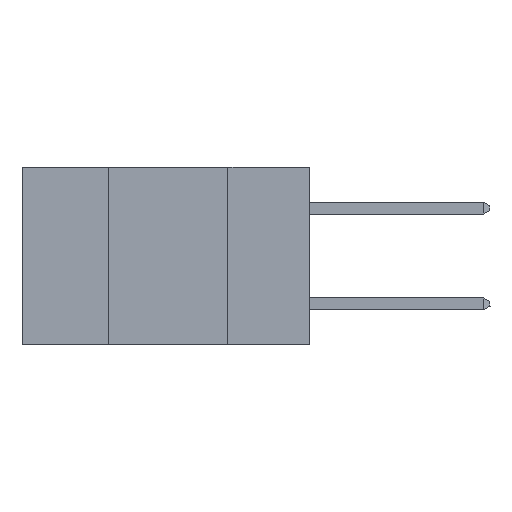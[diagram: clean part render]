
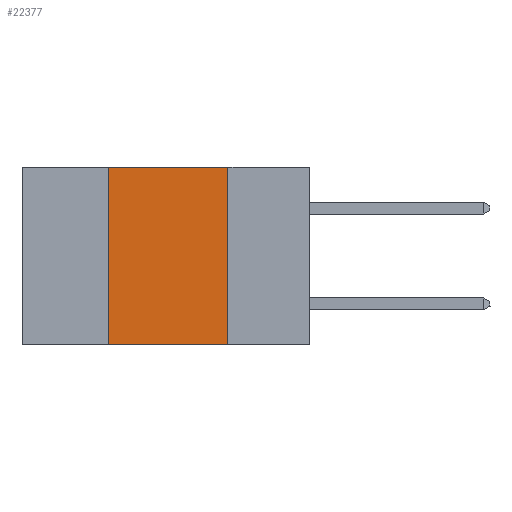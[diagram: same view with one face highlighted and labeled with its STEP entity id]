
A CAD part, left-side view. The second image highlights one B-rep face of the part: STEP entity #22377.
In plain terms, the highlighted planar face has unit normal (-1, 0, 0).
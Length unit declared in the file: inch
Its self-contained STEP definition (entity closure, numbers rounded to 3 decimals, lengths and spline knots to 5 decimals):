
#295 = EDGE_CURVE ( 'NONE', #17158, #25781, #14464, .T. ) ;
#1263 = EDGE_LOOP ( 'NONE', ( #10814, #28822, #29011, #9692 ) ) ;
#1396 = CARTESIAN_POINT ( 'NONE',  ( 0., 0.17, -0.37 ) ) ;
#2312 = VECTOR ( 'NONE', #17650, 39.37008 ) ;
#3037 = AXIS2_PLACEMENT_3D ( 'NONE', #12437, #6831, #18360 ) ;
#5322 = DIRECTION ( 'NONE',  ( 0., -1., 0. ) ) ;
#5806 = LINE ( 'NONE', #28893, #7790 ) ;
#6831 = DIRECTION ( 'NONE',  ( 1., 0., 0. ) ) ;
#7790 = VECTOR ( 'NONE', #18457, 39.37008 ) ;
#9297 = PLANE ( 'NONE',  #3037 ) ;
#9692 = ORIENTED_EDGE ( 'NONE', *, *, #11433, .T. ) ;
#9768 = CARTESIAN_POINT ( 'NONE',  ( 0., 0.6, -0.37 ) ) ;
#10146 = CARTESIAN_POINT ( 'NONE',  ( 0., 0.42, -0.37 ) ) ;
#10175 = CARTESIAN_POINT ( 'NONE',  ( 0., 0.17, 0. ) ) ;
#10814 = ORIENTED_EDGE ( 'NONE', *, *, #295, .F. ) ;
#11433 = EDGE_CURVE ( 'NONE', #31203, #25781, #30678, .T. ) ;
#12437 = CARTESIAN_POINT ( 'NONE',  ( 0., 0.6, 0. ) ) ;
#14464 = LINE ( 'NONE', #10175, #2312 ) ;
#15812 = LINE ( 'NONE', #20394, #26854 ) ;
#17158 = VERTEX_POINT ( 'NONE', #29191 ) ;
#17650 = DIRECTION ( 'NONE',  ( 0., 0., -1. ) ) ;
#18360 = DIRECTION ( 'NONE',  ( 0., 0., -1. ) ) ;
#18442 = EDGE_CURVE ( 'NONE', #31203, #27503, #5806, .T. ) ;
#18457 = DIRECTION ( 'NONE',  ( 0., 0., 1. ) ) ;
#20394 = CARTESIAN_POINT ( 'NONE',  ( 0., 0.6, 0. ) ) ;
#21438 = FACE_OUTER_BOUND ( 'NONE', #1263, .T. ) ;
#22377 = ADVANCED_FACE ( 'NONE', ( #21438 ), #9297, .F. ) ;
#23201 = EDGE_CURVE ( 'NONE', #27503, #17158, #15812, .T. ) ;
#24090 = VECTOR ( 'NONE', #28735, 39.37008 ) ;
#25781 = VERTEX_POINT ( 'NONE', #1396 ) ;
#25930 = CARTESIAN_POINT ( 'NONE',  ( 0., 0.42, 0. ) ) ;
#26854 = VECTOR ( 'NONE', #5322, 39.37008 ) ;
#27503 = VERTEX_POINT ( 'NONE', #25930 ) ;
#28735 = DIRECTION ( 'NONE',  ( 0., -1., 0. ) ) ;
#28822 = ORIENTED_EDGE ( 'NONE', *, *, #23201, .F. ) ;
#28893 = CARTESIAN_POINT ( 'NONE',  ( 0., 0.42, 0. ) ) ;
#29011 = ORIENTED_EDGE ( 'NONE', *, *, #18442, .F. ) ;
#29191 = CARTESIAN_POINT ( 'NONE',  ( 0., 0.17, 0. ) ) ;
#30678 = LINE ( 'NONE', #9768, #24090 ) ;
#31203 = VERTEX_POINT ( 'NONE', #10146 ) ;
